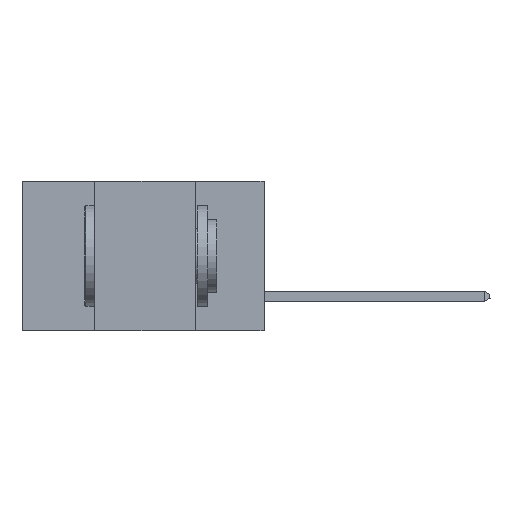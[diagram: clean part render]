
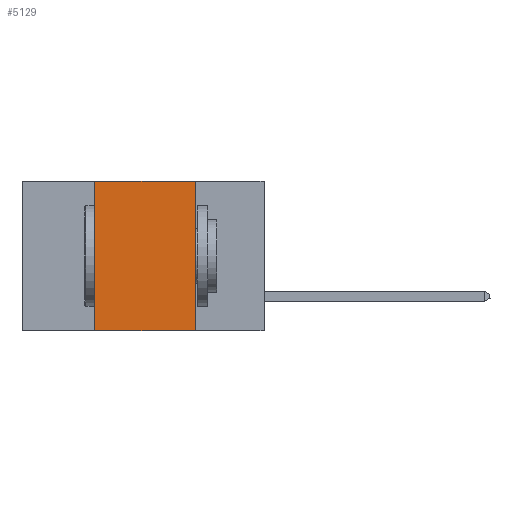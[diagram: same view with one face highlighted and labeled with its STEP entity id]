
A CAD part, left-side view. The second image highlights one B-rep face of the part: STEP entity #5129.
In plain terms, the highlighted planar face has unit normal (-1, 0, 0).
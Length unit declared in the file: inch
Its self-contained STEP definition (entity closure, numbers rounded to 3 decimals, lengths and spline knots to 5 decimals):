
#273 = EDGE_LOOP ( 'NONE', ( #3703, #7749, #27214, #4198 ) ) ;
#855 = VERTEX_POINT ( 'NONE', #17651 ) ;
#964 = CARTESIAN_POINT ( 'NONE',  ( 0., 0.42, 0. ) ) ;
#1258 = DIRECTION ( 'NONE',  ( 0., 0., 1. ) ) ;
#2260 = CARTESIAN_POINT ( 'NONE',  ( 0., 0.17, 0. ) ) ;
#3703 = ORIENTED_EDGE ( 'NONE', *, *, #27883, .F. ) ;
#4198 = ORIENTED_EDGE ( 'NONE', *, *, #22035, .T. ) ;
#5129 = ADVANCED_FACE ( 'NONE', ( #21188 ), #19469, .F. ) ;
#7117 = VECTOR ( 'NONE', #1258, 39.37008 ) ;
#7749 = ORIENTED_EDGE ( 'NONE', *, *, #10628, .F. ) ;
#8367 = CARTESIAN_POINT ( 'NONE',  ( 0., 0.6, -0.37 ) ) ;
#9002 = CARTESIAN_POINT ( 'NONE',  ( 0., 0.6, 0. ) ) ;
#9170 = CARTESIAN_POINT ( 'NONE',  ( 0., 0.17, -0.37 ) ) ;
#9929 = VERTEX_POINT ( 'NONE', #9170 ) ;
#9953 = DIRECTION ( 'NONE',  ( 1., 0., 0. ) ) ;
#10628 = EDGE_CURVE ( 'NONE', #855, #27491, #16662, .T. ) ;
#10750 = DIRECTION ( 'NONE',  ( 0., -1., 0. ) ) ;
#11187 = LINE ( 'NONE', #964, #7117 ) ;
#13038 = AXIS2_PLACEMENT_3D ( 'NONE', #24245, #9953, #19362 ) ;
#14865 = VERTEX_POINT ( 'NONE', #15679 ) ;
#15679 = CARTESIAN_POINT ( 'NONE',  ( 0., 0.42, -0.37 ) ) ;
#16662 = LINE ( 'NONE', #9002, #23336 ) ;
#17062 = DIRECTION ( 'NONE',  ( 0., 0., -1. ) ) ;
#17651 = CARTESIAN_POINT ( 'NONE',  ( 0., 0.42, 0. ) ) ;
#19251 = CARTESIAN_POINT ( 'NONE',  ( 0., 0.17, 0. ) ) ;
#19362 = DIRECTION ( 'NONE',  ( 0., 0., -1. ) ) ;
#19469 = PLANE ( 'NONE',  #13038 ) ;
#19995 = VECTOR ( 'NONE', #10750, 39.37008 ) ;
#20719 = LINE ( 'NONE', #8367, #19995 ) ;
#21188 = FACE_OUTER_BOUND ( 'NONE', #273, .T. ) ;
#22035 = EDGE_CURVE ( 'NONE', #14865, #9929, #20719, .T. ) ;
#22954 = LINE ( 'NONE', #19251, #27768 ) ;
#23336 = VECTOR ( 'NONE', #23354, 39.37008 ) ;
#23354 = DIRECTION ( 'NONE',  ( 0., -1., 0. ) ) ;
#24245 = CARTESIAN_POINT ( 'NONE',  ( 0., 0.6, 0. ) ) ;
#25138 = EDGE_CURVE ( 'NONE', #14865, #855, #11187, .T. ) ;
#27214 = ORIENTED_EDGE ( 'NONE', *, *, #25138, .F. ) ;
#27491 = VERTEX_POINT ( 'NONE', #2260 ) ;
#27768 = VECTOR ( 'NONE', #17062, 39.37008 ) ;
#27883 = EDGE_CURVE ( 'NONE', #27491, #9929, #22954, .T. ) ;
